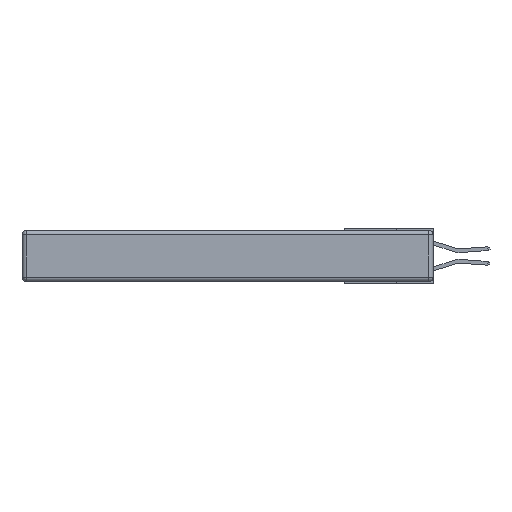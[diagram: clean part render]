
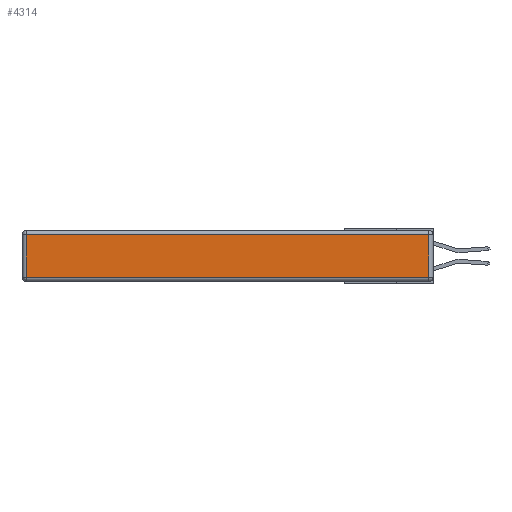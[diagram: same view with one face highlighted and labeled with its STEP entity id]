
A CAD part, left-side view. The second image highlights one B-rep face of the part: STEP entity #4314.
In plain terms, the highlighted planar face has unit normal (-1, 0, 0).
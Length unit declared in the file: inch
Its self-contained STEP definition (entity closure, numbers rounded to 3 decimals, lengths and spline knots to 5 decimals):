
#435 = CARTESIAN_POINT ( 'NONE',  ( 0., 0.03, -0.03 ) ) ;
#1516 = VERTEX_POINT ( 'NONE', #24243 ) ;
#2460 = ORIENTED_EDGE ( 'NONE', *, *, #20201, .T. ) ;
#3769 = DIRECTION ( 'NONE',  ( 0., 0., 1. ) ) ;
#4128 = CARTESIAN_POINT ( 'NONE',  ( 0., 0., -0.313 ) ) ;
#4314 = ADVANCED_FACE ( 'NONE', ( #24606 ), #10885, .T. ) ;
#5035 = DIRECTION ( 'NONE',  ( -1., 0., 0. ) ) ;
#6155 = ORIENTED_EDGE ( 'NONE', *, *, #10592, .T. ) ;
#6793 = CARTESIAN_POINT ( 'NONE',  ( 0., 2.75, -0.03 ) ) ;
#7501 = VECTOR ( 'NONE', #3769, 39.37008 ) ;
#8478 = LINE ( 'NONE', #11685, #7501 ) ;
#8947 = DIRECTION ( 'NONE',  ( 0., 0., 1. ) ) ;
#9754 = CARTESIAN_POINT ( 'NONE',  ( 0., 2.72, -0.343 ) ) ;
#9843 = DIRECTION ( 'NONE',  ( 0., 0., -1. ) ) ;
#10112 = VECTOR ( 'NONE', #9843, 39.37008 ) ;
#10190 = EDGE_LOOP ( 'NONE', ( #2460, #6155, #24049, #17493 ) ) ;
#10592 = EDGE_CURVE ( 'NONE', #1516, #15718, #8478, .T. ) ;
#10822 = DIRECTION ( 'NONE',  ( 0., 1., 0. ) ) ;
#10885 = PLANE ( 'NONE',  #15858 ) ;
#11685 = CARTESIAN_POINT ( 'NONE',  ( 0., 0.03, -0.343 ) ) ;
#12777 = VERTEX_POINT ( 'NONE', #22922 ) ;
#13630 = LINE ( 'NONE', #4128, #15512 ) ;
#15512 = VECTOR ( 'NONE', #16064, 39.37008 ) ;
#15718 = VERTEX_POINT ( 'NONE', #435 ) ;
#15858 = AXIS2_PLACEMENT_3D ( 'NONE', #23135, #5035, #8947 ) ;
#16064 = DIRECTION ( 'NONE',  ( 0., -1., 0. ) ) ;
#16330 = LINE ( 'NONE', #6793, #20971 ) ;
#16599 = EDGE_CURVE ( 'NONE', #15718, #12777, #16330, .T. ) ;
#17493 = ORIENTED_EDGE ( 'NONE', *, *, #21932, .T. ) ;
#18819 = LINE ( 'NONE', #9754, #10112 ) ;
#20201 = EDGE_CURVE ( 'NONE', #22828, #1516, #13630, .T. ) ;
#20971 = VECTOR ( 'NONE', #10822, 39.37008 ) ;
#21864 = CARTESIAN_POINT ( 'NONE',  ( 0., 2.72, -0.313 ) ) ;
#21932 = EDGE_CURVE ( 'NONE', #12777, #22828, #18819, .T. ) ;
#22828 = VERTEX_POINT ( 'NONE', #21864 ) ;
#22922 = CARTESIAN_POINT ( 'NONE',  ( 0., 2.72, -0.03 ) ) ;
#23135 = CARTESIAN_POINT ( 'NONE',  ( 0., 0., -0.343 ) ) ;
#24049 = ORIENTED_EDGE ( 'NONE', *, *, #16599, .T. ) ;
#24243 = CARTESIAN_POINT ( 'NONE',  ( 0., 0.03, -0.313 ) ) ;
#24606 = FACE_OUTER_BOUND ( 'NONE', #10190, .T. ) ;
